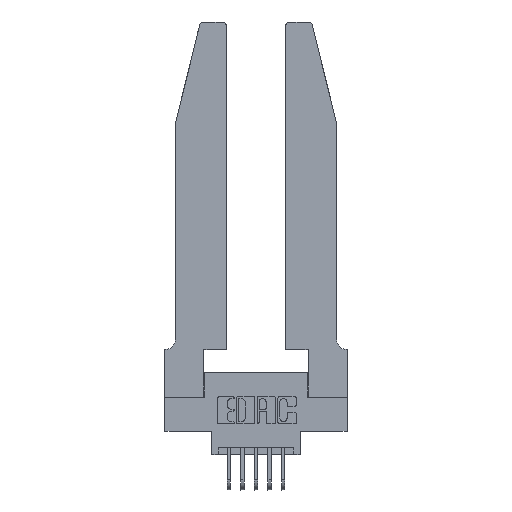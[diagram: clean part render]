
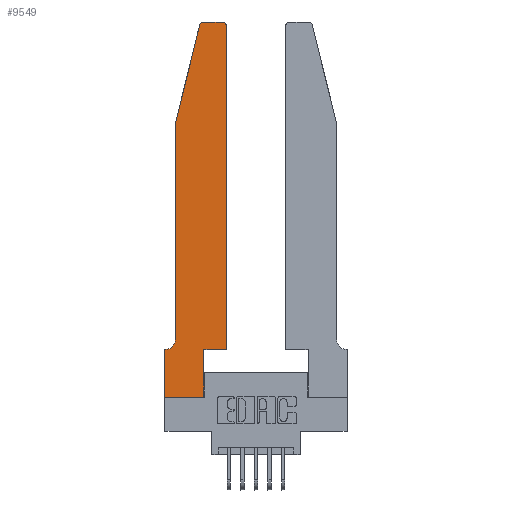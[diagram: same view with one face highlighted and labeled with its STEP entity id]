
A CAD part, top view. The second image highlights one B-rep face of the part: STEP entity #9549.
In plain terms, the highlighted planar face has unit normal (0, 0, 1).
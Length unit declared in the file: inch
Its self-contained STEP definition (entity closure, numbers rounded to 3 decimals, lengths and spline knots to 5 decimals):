
#81 = CIRCLE ( 'NONE', #12375, 0.03 ) ;
#213 = LINE ( 'NONE', #9617, #8814 ) ;
#405 = ORIENTED_EDGE ( 'NONE', *, *, #9209, .T. ) ;
#431 = DIRECTION ( 'NONE',  ( 0., -1., 0. ) ) ;
#704 = VECTOR ( 'NONE', #1576, 39.37008 ) ;
#782 = VERTEX_POINT ( 'NONE', #9069 ) ;
#1453 = VECTOR ( 'NONE', #7224, 39.37008 ) ;
#1497 = VERTEX_POINT ( 'NONE', #4275 ) ;
#1506 = CARTESIAN_POINT ( 'NONE',  ( 0.0755, 2., 0.37 ) ) ;
#1576 = DIRECTION ( 'NONE',  ( -0.239, -0.971, 0. ) ) ;
#1684 = EDGE_CURVE ( 'NONE', #2203, #12755, #12563, .T. ) ;
#1766 = LINE ( 'NONE', #1506, #12599 ) ;
#1927 = EDGE_LOOP ( 'NONE', ( #10375, #4337, #6089, #11134, #11379, #12571, #8333, #11203, #12455, #13561, #405, #12643 ) ) ;
#1940 = DIRECTION ( 'NONE',  ( 0., 0., 1. ) ) ;
#2203 = VERTEX_POINT ( 'NONE', #2771 ) ;
#2352 = DIRECTION ( 'NONE',  ( -1., 0., 0. ) ) ;
#2578 = VERTEX_POINT ( 'NONE', #3668 ) ;
#2690 = LINE ( 'NONE', #12419, #8023 ) ;
#2771 = CARTESIAN_POINT ( 'NONE',  ( 0., 0., 0.37 ) ) ;
#2846 = DIRECTION ( 'NONE',  ( 1., 0., 0. ) ) ;
#3131 = EDGE_CURVE ( 'NONE', #12496, #10980, #11420, .T. ) ;
#3203 = VECTOR ( 'NONE', #2352, 39.37008 ) ;
#3251 = CARTESIAN_POINT ( 'NONE',  ( 0.0755, 0.35, 0.37 ) ) ;
#3374 = CARTESIAN_POINT ( 'NONE',  ( 0.2865, 0.35, 0.37 ) ) ;
#3668 = CARTESIAN_POINT ( 'NONE',  ( 0.4505, 0.35, 0.37 ) ) ;
#3959 = EDGE_CURVE ( 'NONE', #10934, #11336, #81, .T. ) ;
#4275 = CARTESIAN_POINT ( 'NONE',  ( 0., 0.35, 0.37 ) ) ;
#4337 = ORIENTED_EDGE ( 'NONE', *, *, #3959, .T. ) ;
#4398 = CARTESIAN_POINT ( 'NONE',  ( 0., 0., 0.37 ) ) ;
#4508 = CIRCLE ( 'NONE', #5955, 0.07 ) ;
#4641 = AXIS2_PLACEMENT_3D ( 'NONE', #10838, #4649, #11830 ) ;
#4649 = DIRECTION ( 'NONE',  ( 0., 0., 1. ) ) ;
#4706 = VECTOR ( 'NONE', #7959, 39.37008 ) ;
#4893 = CARTESIAN_POINT ( 'NONE',  ( 0.2865, 0., 0.37 ) ) ;
#5032 = CARTESIAN_POINT ( 'NONE',  ( 0., 0.35, 0.37 ) ) ;
#5209 = VERTEX_POINT ( 'NONE', #6344 ) ;
#5258 = VECTOR ( 'NONE', #13663, 39.37008 ) ;
#5473 = CARTESIAN_POINT ( 'NONE',  ( 0.25487, 2.72718, 0.37 ) ) ;
#5769 = EDGE_CURVE ( 'NONE', #12755, #8702, #12314, .T. ) ;
#5947 = EDGE_CURVE ( 'NONE', #5209, #1497, #13443, .T. ) ;
#5955 = AXIS2_PLACEMENT_3D ( 'NONE', #12570, #6470, #13606 ) ;
#6089 = ORIENTED_EDGE ( 'NONE', *, *, #7666, .T. ) ;
#6202 = CARTESIAN_POINT ( 'NONE',  ( 0.2865, 0.35, 0.37 ) ) ;
#6344 = CARTESIAN_POINT ( 'NONE',  ( 0.0055, 0.35, 0.37 ) ) ;
#6370 = VERTEX_POINT ( 'NONE', #10566 ) ;
#6470 = DIRECTION ( 'NONE',  ( 0., 0., -1. ) ) ;
#7000 = CARTESIAN_POINT ( 'NONE',  ( 0.0755, 2., 0.37 ) ) ;
#7224 = DIRECTION ( 'NONE',  ( 0., 1., 0. ) ) ;
#7651 = CARTESIAN_POINT ( 'NONE',  ( 0.4505, 2.72, 0.37 ) ) ;
#7666 = EDGE_CURVE ( 'NONE', #11336, #6370, #9243, .T. ) ;
#7698 = VECTOR ( 'NONE', #11584, 39.37008 ) ;
#7959 = DIRECTION ( 'NONE',  ( 1., 0., 0. ) ) ;
#8008 = FACE_OUTER_BOUND ( 'NONE', #1927, .T. ) ;
#8023 = VECTOR ( 'NONE', #13458, 39.37008 ) ;
#8141 = PLANE ( 'NONE',  #10058 ) ;
#8333 = ORIENTED_EDGE ( 'NONE', *, *, #9051, .T. ) ;
#8337 = CARTESIAN_POINT ( 'NONE',  ( 0.284, 2.72, 0.37 ) ) ;
#8627 = DIRECTION ( 'NONE',  ( 0., 1., 0. ) ) ;
#8702 = VERTEX_POINT ( 'NONE', #3374 ) ;
#8735 = CARTESIAN_POINT ( 'NONE',  ( 0.284, 2.75, 0.37 ) ) ;
#8814 = VECTOR ( 'NONE', #8627, 39.37008 ) ;
#9051 = EDGE_CURVE ( 'NONE', #1497, #2203, #2690, .T. ) ;
#9069 = CARTESIAN_POINT ( 'NONE',  ( 0.0755, 0.42, 0.37 ) ) ;
#9163 = DIRECTION ( 'NONE',  ( 0., 0., 1. ) ) ;
#9209 = EDGE_CURVE ( 'NONE', #2578, #12496, #213, .T. ) ;
#9243 = LINE ( 'NONE', #7000, #704 ) ;
#9361 = DIRECTION ( 'NONE',  ( 1., 0., 0. ) ) ;
#9549 = ADVANCED_FACE ( 'NONE', ( #8008 ), #8141, .T. ) ;
#9617 = CARTESIAN_POINT ( 'NONE',  ( 0.4505, 0.35, 0.37 ) ) ;
#9782 = EDGE_CURVE ( 'NONE', #10980, #10934, #11831, .T. ) ;
#10058 = AXIS2_PLACEMENT_3D ( 'NONE', #5032, #9163, #2846 ) ;
#10362 = EDGE_CURVE ( 'NONE', #8702, #2578, #13127, .T. ) ;
#10375 = ORIENTED_EDGE ( 'NONE', *, *, #9782, .T. ) ;
#10566 = CARTESIAN_POINT ( 'NONE',  ( 0.0755, 2., 0.37 ) ) ;
#10838 = CARTESIAN_POINT ( 'NONE',  ( 0.4205, 2.72, 0.37 ) ) ;
#10934 = VERTEX_POINT ( 'NONE', #8735 ) ;
#10980 = VERTEX_POINT ( 'NONE', #11853 ) ;
#11134 = ORIENTED_EDGE ( 'NONE', *, *, #11541, .T. ) ;
#11203 = ORIENTED_EDGE ( 'NONE', *, *, #1684, .T. ) ;
#11336 = VERTEX_POINT ( 'NONE', #5473 ) ;
#11379 = ORIENTED_EDGE ( 'NONE', *, *, #13661, .T. ) ;
#11420 = CIRCLE ( 'NONE', #4641, 0.03 ) ;
#11541 = EDGE_CURVE ( 'NONE', #6370, #782, #1766, .T. ) ;
#11584 = DIRECTION ( 'NONE',  ( -1., 0., 0. ) ) ;
#11830 = DIRECTION ( 'NONE',  ( 1., 0., 0. ) ) ;
#11831 = LINE ( 'NONE', #12825, #3203 ) ;
#11853 = CARTESIAN_POINT ( 'NONE',  ( 0.4205, 2.75, 0.37 ) ) ;
#12314 = LINE ( 'NONE', #6202, #1453 ) ;
#12375 = AXIS2_PLACEMENT_3D ( 'NONE', #8337, #1940, #9361 ) ;
#12419 = CARTESIAN_POINT ( 'NONE',  ( 0., 0., 0.37 ) ) ;
#12455 = ORIENTED_EDGE ( 'NONE', *, *, #5769, .T. ) ;
#12496 = VERTEX_POINT ( 'NONE', #7651 ) ;
#12563 = LINE ( 'NONE', #4398, #4706 ) ;
#12570 = CARTESIAN_POINT ( 'NONE',  ( 0.0055, 0.42, 0.37 ) ) ;
#12571 = ORIENTED_EDGE ( 'NONE', *, *, #5947, .T. ) ;
#12599 = VECTOR ( 'NONE', #431, 39.37008 ) ;
#12621 = CARTESIAN_POINT ( 'NONE',  ( 0.4505, 0.35, 0.37 ) ) ;
#12643 = ORIENTED_EDGE ( 'NONE', *, *, #3131, .T. ) ;
#12755 = VERTEX_POINT ( 'NONE', #4893 ) ;
#12825 = CARTESIAN_POINT ( 'NONE',  ( 0.2605, 2.75, 0.37 ) ) ;
#13127 = LINE ( 'NONE', #12621, #5258 ) ;
#13443 = LINE ( 'NONE', #3251, #7698 ) ;
#13458 = DIRECTION ( 'NONE',  ( 0., -1., 0. ) ) ;
#13561 = ORIENTED_EDGE ( 'NONE', *, *, #10362, .T. ) ;
#13606 = DIRECTION ( 'NONE',  ( -1., 0., 0. ) ) ;
#13661 = EDGE_CURVE ( 'NONE', #782, #5209, #4508, .T. ) ;
#13663 = DIRECTION ( 'NONE',  ( 1., 0., 0. ) ) ;
